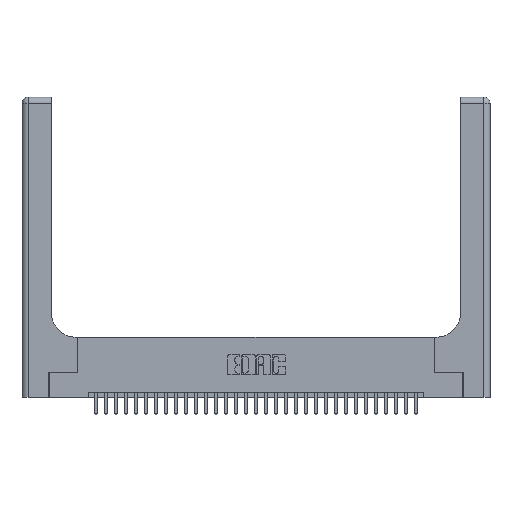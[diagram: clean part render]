
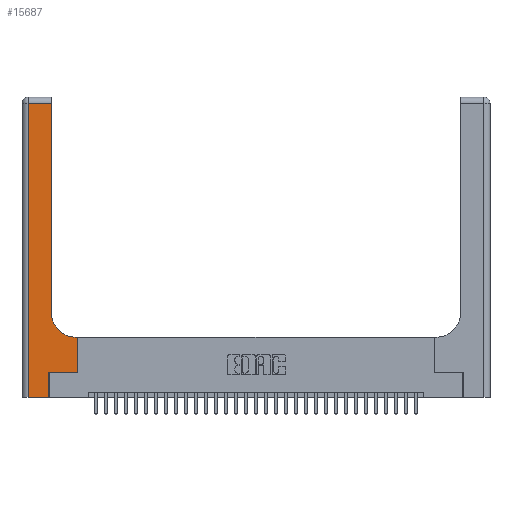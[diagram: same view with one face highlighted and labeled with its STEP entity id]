
A CAD part, top view. The second image highlights one B-rep face of the part: STEP entity #15687.
In plain terms, the highlighted planar face has unit normal (0, 0, 1).
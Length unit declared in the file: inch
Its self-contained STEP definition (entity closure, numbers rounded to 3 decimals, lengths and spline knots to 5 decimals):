
#268 = CARTESIAN_POINT ( 'NONE',  ( 0.5585, 0.6, 0.37 ) ) ;
#995 = CARTESIAN_POINT ( 'NONE',  ( 0.06, 3., 0.37 ) ) ;
#1923 = LINE ( 'NONE', #16220, #14437 ) ;
#2000 = ORIENTED_EDGE ( 'NONE', *, *, #15067, .T. ) ;
#2075 = VECTOR ( 'NONE', #30660, 39.37008 ) ;
#2664 = DIRECTION ( 'NONE',  ( -1., 0., 0. ) ) ;
#2905 = PLANE ( 'NONE',  #30507 ) ;
#3326 = VECTOR ( 'NONE', #9542, 39.37008 ) ;
#4465 = VECTOR ( 'NONE', #29067, 39.37008 ) ;
#5077 = VERTEX_POINT ( 'NONE', #21032 ) ;
#5088 = DIRECTION ( 'NONE',  ( 0., 0., -1. ) ) ;
#5162 = ORIENTED_EDGE ( 'NONE', *, *, #30837, .T. ) ;
#5252 = CARTESIAN_POINT ( 'NONE',  ( 0.5585, 0.25, 0.37 ) ) ;
#6457 = LINE ( 'NONE', #6640, #27270 ) ;
#6640 = CARTESIAN_POINT ( 'NONE',  ( 0.269, 0., 0.37 ) ) ;
#6760 = ORIENTED_EDGE ( 'NONE', *, *, #11371, .T. ) ;
#6926 = ORIENTED_EDGE ( 'NONE', *, *, #31980, .T. ) ;
#7004 = ORIENTED_EDGE ( 'NONE', *, *, #17090, .T. ) ;
#7731 = VERTEX_POINT ( 'NONE', #19295 ) ;
#7940 = LINE ( 'NONE', #13117, #2075 ) ;
#8139 = CARTESIAN_POINT ( 'NONE',  ( 0.269, 0.25, 0.37 ) ) ;
#8874 = VERTEX_POINT ( 'NONE', #26807 ) ;
#9542 = DIRECTION ( 'NONE',  ( 0., 1., 0. ) ) ;
#9765 = ORIENTED_EDGE ( 'NONE', *, *, #26317, .T. ) ;
#10002 = LINE ( 'NONE', #27074, #15885 ) ;
#10441 = CARTESIAN_POINT ( 'NONE',  ( 0., 3., 0.37 ) ) ;
#10550 = CIRCLE ( 'NONE', #18460, 0.25 ) ;
#11041 = EDGE_CURVE ( 'NONE', #28212, #5077, #10550, .T. ) ;
#11217 = VERTEX_POINT ( 'NONE', #8139 ) ;
#11371 = EDGE_CURVE ( 'NONE', #8874, #12974, #1923, .T. ) ;
#12591 = ORIENTED_EDGE ( 'NONE', *, *, #24390, .T. ) ;
#12961 = DIRECTION ( 'NONE',  ( -1., 0., 0. ) ) ;
#12974 = VERTEX_POINT ( 'NONE', #30177 ) ;
#13117 = CARTESIAN_POINT ( 'NONE',  ( 0., 0., 0.37 ) ) ;
#14153 = VECTOR ( 'NONE', #2664, 39.37008 ) ;
#14313 = ORIENTED_EDGE ( 'NONE', *, *, #23592, .T. ) ;
#14437 = VECTOR ( 'NONE', #18757, 39.37008 ) ;
#14578 = CARTESIAN_POINT ( 'NONE',  ( 0.2915, 3., 0.37 ) ) ;
#14931 = LINE ( 'NONE', #15130, #14153 ) ;
#15067 = EDGE_CURVE ( 'NONE', #7731, #29494, #7940, .T. ) ;
#15130 = CARTESIAN_POINT ( 'NONE',  ( 0.2915, 0.6, 0.37 ) ) ;
#15687 = ADVANCED_FACE ( 'NONE', ( #17305 ), #2905, .F. ) ;
#15885 = VECTOR ( 'NONE', #19600, 39.37008 ) ;
#16220 = CARTESIAN_POINT ( 'NONE',  ( 0., 2.94, 0.37 ) ) ;
#17090 = EDGE_CURVE ( 'NONE', #12974, #7731, #28223, .T. ) ;
#17305 = FACE_OUTER_BOUND ( 'NONE', #31952, .T. ) ;
#17415 = LINE ( 'NONE', #14578, #3326 ) ;
#18460 = AXIS2_PLACEMENT_3D ( 'NONE', #20104, #5088, #22643 ) ;
#18493 = DIRECTION ( 'NONE',  ( 0., -1., 0. ) ) ;
#18757 = DIRECTION ( 'NONE',  ( -1., 0., 0. ) ) ;
#19295 = CARTESIAN_POINT ( 'NONE',  ( 0.06, 0., 0.37 ) ) ;
#19600 = DIRECTION ( 'NONE',  ( 1., 0., 0. ) ) ;
#20104 = CARTESIAN_POINT ( 'NONE',  ( 0.5415, 0.85, 0.37 ) ) ;
#21032 = CARTESIAN_POINT ( 'NONE',  ( 0.2915, 0.85, 0.37 ) ) ;
#22347 = VECTOR ( 'NONE', #18493, 39.37008 ) ;
#22643 = DIRECTION ( 'NONE',  ( 1., 0., 0. ) ) ;
#23053 = ORIENTED_EDGE ( 'NONE', *, *, #11041, .T. ) ;
#23592 = EDGE_CURVE ( 'NONE', #29494, #11217, #6457, .T. ) ;
#24052 = CARTESIAN_POINT ( 'NONE',  ( 0.5585, 0.25, 0.37 ) ) ;
#24213 = DIRECTION ( 'NONE',  ( 0., 1., 0. ) ) ;
#24390 = EDGE_CURVE ( 'NONE', #5077, #8874, #17415, .T. ) ;
#24486 = LINE ( 'NONE', #24052, #4465 ) ;
#26317 = EDGE_CURVE ( 'NONE', #26359, #28212, #14931, .T. ) ;
#26359 = VERTEX_POINT ( 'NONE', #268 ) ;
#26421 = CARTESIAN_POINT ( 'NONE',  ( 0.5415, 0.6, 0.37 ) ) ;
#26807 = CARTESIAN_POINT ( 'NONE',  ( 0.2915, 2.94, 0.37 ) ) ;
#27074 = CARTESIAN_POINT ( 'NONE',  ( 0.269, 0.25, 0.37 ) ) ;
#27270 = VECTOR ( 'NONE', #24213, 39.37008 ) ;
#28014 = DIRECTION ( 'NONE',  ( 0., 0., -1. ) ) ;
#28212 = VERTEX_POINT ( 'NONE', #26421 ) ;
#28223 = LINE ( 'NONE', #995, #22347 ) ;
#29067 = DIRECTION ( 'NONE',  ( 0., 1., 0. ) ) ;
#29312 = CARTESIAN_POINT ( 'NONE',  ( 0.269, 0., 0.37 ) ) ;
#29494 = VERTEX_POINT ( 'NONE', #29312 ) ;
#30177 = CARTESIAN_POINT ( 'NONE',  ( 0.06, 2.94, 0.37 ) ) ;
#30452 = VERTEX_POINT ( 'NONE', #5252 ) ;
#30507 = AXIS2_PLACEMENT_3D ( 'NONE', #10441, #28014, #12961 ) ;
#30660 = DIRECTION ( 'NONE',  ( 1., 0., 0. ) ) ;
#30837 = EDGE_CURVE ( 'NONE', #11217, #30452, #10002, .T. ) ;
#31952 = EDGE_LOOP ( 'NONE', ( #12591, #6760, #7004, #2000, #14313, #5162, #6926, #9765, #23053 ) ) ;
#31980 = EDGE_CURVE ( 'NONE', #30452, #26359, #24486, .T. ) ;
